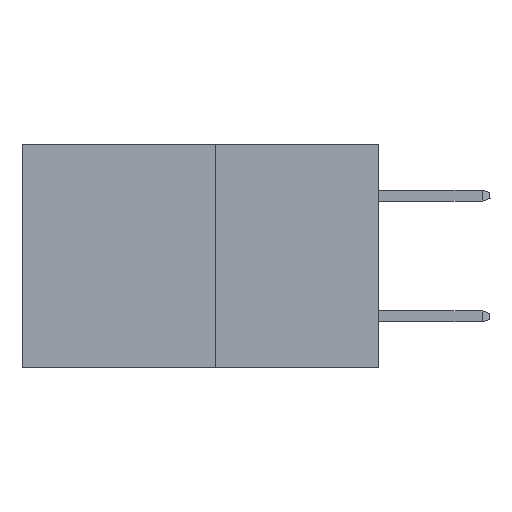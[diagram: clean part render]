
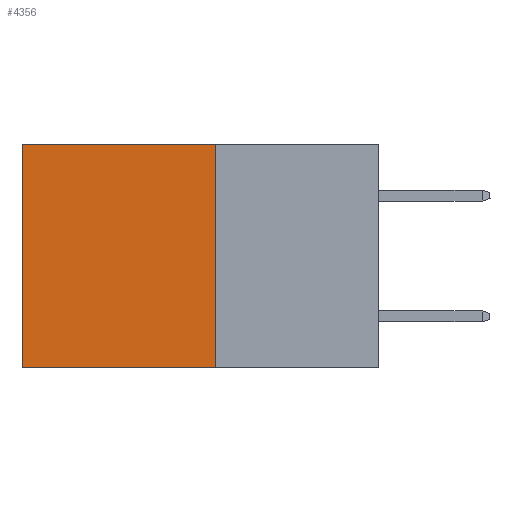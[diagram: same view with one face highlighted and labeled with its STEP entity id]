
A CAD part, left-side view. The second image highlights one B-rep face of the part: STEP entity #4356.
In plain terms, the highlighted planar face has unit normal (-1, 0, 0).
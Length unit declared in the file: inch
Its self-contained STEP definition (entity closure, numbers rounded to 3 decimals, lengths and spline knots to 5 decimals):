
#911 = DIRECTION ( 'NONE',  ( 0., 1., 0. ) ) ;
#2097 = VECTOR ( 'NONE', #9735, 39.37008 ) ;
#2678 = LINE ( 'NONE', #18834, #2097 ) ;
#2748 = ORIENTED_EDGE ( 'NONE', *, *, #16374, .F. ) ;
#3325 = EDGE_CURVE ( 'NONE', #12282, #3945, #4576, .T. ) ;
#3945 = VERTEX_POINT ( 'NONE', #9048 ) ;
#4356 = ADVANCED_FACE ( 'NONE', ( #7204 ), #11178, .F. ) ;
#4576 = LINE ( 'NONE', #6830, #9332 ) ;
#5742 = ORIENTED_EDGE ( 'NONE', *, *, #8284, .F. ) ;
#5973 = ORIENTED_EDGE ( 'NONE', *, *, #3325, .T. ) ;
#6397 = VECTOR ( 'NONE', #6417, 39.37008 ) ;
#6417 = DIRECTION ( 'NONE',  ( 0., 0., -1. ) ) ;
#6746 = LINE ( 'NONE', #9966, #15846 ) ;
#6830 = CARTESIAN_POINT ( 'NONE',  ( 0.277, 0.27, 0. ) ) ;
#7204 = FACE_OUTER_BOUND ( 'NONE', #9152, .T. ) ;
#7225 = CARTESIAN_POINT ( 'NONE',  ( 0.277, 0.27, -0.37 ) ) ;
#7370 = CARTESIAN_POINT ( 'NONE',  ( 0.277, 0.27, 0. ) ) ;
#8284 = EDGE_CURVE ( 'NONE', #17545, #16547, #6746, .T. ) ;
#9048 = CARTESIAN_POINT ( 'NONE',  ( 0.277, 0.59, 0. ) ) ;
#9152 = EDGE_LOOP ( 'NONE', ( #16506, #5742, #2748, #5973 ) ) ;
#9332 = VECTOR ( 'NONE', #9582, 39.37008 ) ;
#9582 = DIRECTION ( 'NONE',  ( 0., 1., 0. ) ) ;
#9735 = DIRECTION ( 'NONE',  ( 0., 0., -1. ) ) ;
#9966 = CARTESIAN_POINT ( 'NONE',  ( 0.277, 0.27, -0.37 ) ) ;
#10356 = CARTESIAN_POINT ( 'NONE',  ( 0.277, 0.59, -0.37 ) ) ;
#11178 = PLANE ( 'NONE',  #20203 ) ;
#11305 = CARTESIAN_POINT ( 'NONE',  ( 0.277, 0.27, -0.37 ) ) ;
#11330 = DIRECTION ( 'NONE',  ( 1., 0., 0. ) ) ;
#12282 = VERTEX_POINT ( 'NONE', #7370 ) ;
#13638 = CARTESIAN_POINT ( 'NONE',  ( 0.277, 0.27, -0.37 ) ) ;
#15306 = EDGE_CURVE ( 'NONE', #3945, #16547, #2678, .T. ) ;
#15846 = VECTOR ( 'NONE', #911, 39.37008 ) ;
#16374 = EDGE_CURVE ( 'NONE', #12282, #17545, #23012, .T. ) ;
#16506 = ORIENTED_EDGE ( 'NONE', *, *, #15306, .T. ) ;
#16547 = VERTEX_POINT ( 'NONE', #10356 ) ;
#17545 = VERTEX_POINT ( 'NONE', #7225 ) ;
#18834 = CARTESIAN_POINT ( 'NONE',  ( 0.277, 0.59, -0.37 ) ) ;
#20203 = AXIS2_PLACEMENT_3D ( 'NONE', #11305, #11330, #20889 ) ;
#20889 = DIRECTION ( 'NONE',  ( 0., 0., -1. ) ) ;
#23012 = LINE ( 'NONE', #13638, #6397 ) ;
